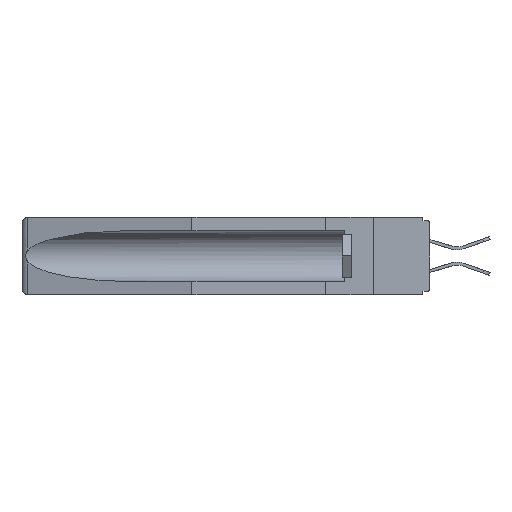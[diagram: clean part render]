
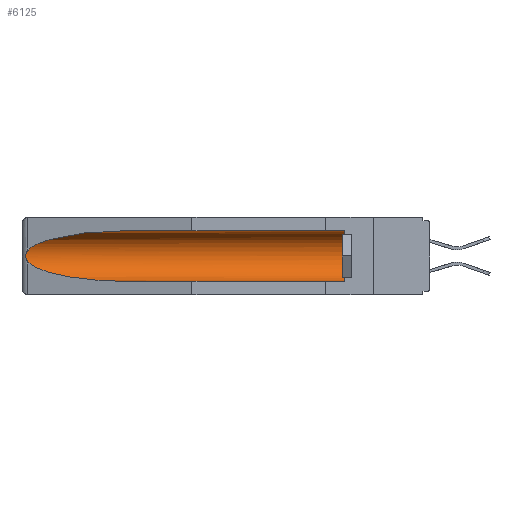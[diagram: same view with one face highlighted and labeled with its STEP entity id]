
A CAD part, left-side view. The second image highlights one B-rep face of the part: STEP entity #6125.
In plain terms, the highlighted cylindrical face has radius 2.857 mm (diameter 5.715 mm), a partial arc.
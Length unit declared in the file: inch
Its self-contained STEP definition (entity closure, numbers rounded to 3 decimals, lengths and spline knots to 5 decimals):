
#260 = DIRECTION ( 'NONE',  ( 0., -1., 0. ) ) ;
#384 = CARTESIAN_POINT ( 'NONE',  ( 0.2673, 1.53269, -0.17917 ) ) ;
#466 = CARTESIAN_POINT ( 'NONE',  ( 0.26654, 1.53092, -0.15636 ) ) ;
#1250 = FACE_OUTER_BOUND ( 'NONE', #13368, .T. ) ;
#1623 = CARTESIAN_POINT ( 'NONE',  ( 0.155, 1.07973, -0.284 ) ) ;
#1814 = DIRECTION ( 'NONE',  ( 0., 0., 1. ) ) ;
#2323 = ORIENTED_EDGE ( 'NONE', *, *, #17232, .T. ) ;
#2584 = VERTEX_POINT ( 'NONE', #4091 ) ;
#2916 = VERTEX_POINT ( 'NONE', #6072 ) ;
#3386 = CARTESIAN_POINT ( 'NONE',  ( 0.21114, 1.30732, -0.284 ) ) ;
#3603 = DIRECTION ( 'NONE',  ( 0., 0., 1. ) ) ;
#3853 = CARTESIAN_POINT ( 'NONE',  ( 0.155, -0.30754, -0.284 ) ) ;
#3909 = VERTEX_POINT ( 'NONE', #11523 ) ;
#3925 = CARTESIAN_POINT ( 'NONE',  ( 0.26537, 1.52718, -0.19328 ) ) ;
#3956 =( BOUNDED_CURVE ( )  B_SPLINE_CURVE ( 3, ( #19397, #8962, #3386, #1623 ),
 .UNSPECIFIED., .F., .F. ) 
 B_SPLINE_CURVE_WITH_KNOTS ( ( 4, 4 ),
 ( 0.1948, 1.5708 ),
 .UNSPECIFIED. ) 
 CURVE ( )  GEOMETRIC_REPRESENTATION_ITEM ( )  RATIONAL_B_SPLINE_CURVE ( ( 1., 0.848, 0.848, 1. ) ) 
 REPRESENTATION_ITEM ( '' )  );
#4091 = CARTESIAN_POINT ( 'NONE',  ( 0.155, 1.07973, -0.284 ) ) ;
#4269 = ORIENTED_EDGE ( 'NONE', *, *, #9168, .T. ) ;
#4898 =( BOUNDED_CURVE ( )  B_SPLINE_CURVE ( 3, ( #15446, #9913, #10280, #8552 ),
 .UNSPECIFIED., .F., .F. ) 
 B_SPLINE_CURVE_WITH_KNOTS ( ( 4, 4 ),
 ( 4.71239, 6.08839 ),
 .UNSPECIFIED. ) 
 CURVE ( )  GEOMETRIC_REPRESENTATION_ITEM ( )  RATIONAL_B_SPLINE_CURVE ( ( 1., 0.848, 0.848, 1. ) ) 
 REPRESENTATION_ITEM ( '' )  );
#5286 = EDGE_CURVE ( 'NONE', #3909, #11014, #4898, .T. ) ;
#6072 = CARTESIAN_POINT ( 'NONE',  ( 0.155, 0.126, -0.059 ) ) ;
#6125 = ADVANCED_FACE ( 'NONE', ( #1250 ), #17048, .F. ) ;
#6933 = ORIENTED_EDGE ( 'NONE', *, *, #10103, .T. ) ;
#7163 = CARTESIAN_POINT ( 'NONE',  ( 0.155, 0.126, -0.1715 ) ) ;
#7302 = AXIS2_PLACEMENT_3D ( 'NONE', #14113, #8639, #3603 ) ;
#7530 = CARTESIAN_POINT ( 'NONE',  ( 0.26537, 1.52718, -0.19328 ) ) ;
#7785 = VECTOR ( 'NONE', #19614, 39.37008 ) ;
#7854 = CIRCLE ( 'NONE', #18884, 0.1125 ) ;
#8095 = VERTEX_POINT ( 'NONE', #19361 ) ;
#8552 = CARTESIAN_POINT ( 'NONE',  ( 0.26537, 1.52718, -0.14972 ) ) ;
#8639 = DIRECTION ( 'NONE',  ( 0., 1., 0. ) ) ;
#8882 = VECTOR ( 'NONE', #12356, 39.37008 ) ;
#8962 = CARTESIAN_POINT ( 'NONE',  ( 0.25451, 1.48313, -0.24835 ) ) ;
#9168 = EDGE_CURVE ( 'NONE', #8095, #2916, #7854, .T. ) ;
#9784 = ORIENTED_EDGE ( 'NONE', *, *, #10204, .F. ) ;
#9913 = CARTESIAN_POINT ( 'NONE',  ( 0.21114, 1.30732, -0.059 ) ) ;
#10103 = EDGE_CURVE ( 'NONE', #2916, #3909, #18140, .T. ) ;
#10204 = EDGE_CURVE ( 'NONE', #8095, #2584, #13738, .T. ) ;
#10280 = CARTESIAN_POINT ( 'NONE',  ( 0.25451, 1.48313, -0.09465 ) ) ;
#10345 = B_SPLINE_CURVE_WITH_KNOTS ( 'NONE', 3,
 ( #15952, #10852, #466, #14444, #17869, #21382, #384, #17945, #12610, #7530 ),
 .UNSPECIFIED., .F., .F.,
 ( 4, 2, 2, 2, 4 ),
 ( 0., 0.00029, 0.00058, 0.00087, 0.00117 ),
 .UNSPECIFIED. ) ;
#10852 = CARTESIAN_POINT ( 'NONE',  ( 0.26597, 1.52961, -0.15275 ) ) ;
#11014 = VERTEX_POINT ( 'NONE', #11791 ) ;
#11523 = CARTESIAN_POINT ( 'NONE',  ( 0.155, 1.07973, -0.059 ) ) ;
#11791 = CARTESIAN_POINT ( 'NONE',  ( 0.26537, 1.52718, -0.14972 ) ) ;
#12356 = DIRECTION ( 'NONE',  ( 0., 1., 0. ) ) ;
#12610 = CARTESIAN_POINT ( 'NONE',  ( 0.26597, 1.5296, -0.19026 ) ) ;
#13368 = EDGE_LOOP ( 'NONE', ( #18874, #2323, #14713, #9784, #4269, #6933 ) ) ;
#13738 = LINE ( 'NONE', #3853, #7785 ) ;
#13969 = CARTESIAN_POINT ( 'NONE',  ( 0.155, -0.30754, -0.059 ) ) ;
#14113 = CARTESIAN_POINT ( 'NONE',  ( 0.155, -0.30754, -0.1715 ) ) ;
#14444 = CARTESIAN_POINT ( 'NONE',  ( 0.2673, 1.5327, -0.16383 ) ) ;
#14623 = EDGE_CURVE ( 'NONE', #20511, #2584, #3956, .T. ) ;
#14713 = ORIENTED_EDGE ( 'NONE', *, *, #14623, .T. ) ;
#15446 = CARTESIAN_POINT ( 'NONE',  ( 0.155, 1.07973, -0.059 ) ) ;
#15952 = CARTESIAN_POINT ( 'NONE',  ( 0.26537, 1.52718, -0.14972 ) ) ;
#17048 = CYLINDRICAL_SURFACE ( 'NONE', #7302, 0.1125 ) ;
#17232 = EDGE_CURVE ( 'NONE', #11014, #20511, #10345, .T. ) ;
#17869 = CARTESIAN_POINT ( 'NONE',  ( 0.2675, 1.53308, -0.16763 ) ) ;
#17945 = CARTESIAN_POINT ( 'NONE',  ( 0.26655, 1.53094, -0.18657 ) ) ;
#18140 = LINE ( 'NONE', #13969, #8882 ) ;
#18874 = ORIENTED_EDGE ( 'NONE', *, *, #5286, .T. ) ;
#18884 = AXIS2_PLACEMENT_3D ( 'NONE', #7163, #260, #1814 ) ;
#19361 = CARTESIAN_POINT ( 'NONE',  ( 0.155, 0.126, -0.284 ) ) ;
#19397 = CARTESIAN_POINT ( 'NONE',  ( 0.26537, 1.52718, -0.19328 ) ) ;
#19614 = DIRECTION ( 'NONE',  ( 0., 1., 0. ) ) ;
#20511 = VERTEX_POINT ( 'NONE', #3925 ) ;
#21382 = CARTESIAN_POINT ( 'NONE',  ( 0.2675, 1.53308, -0.17534 ) ) ;
